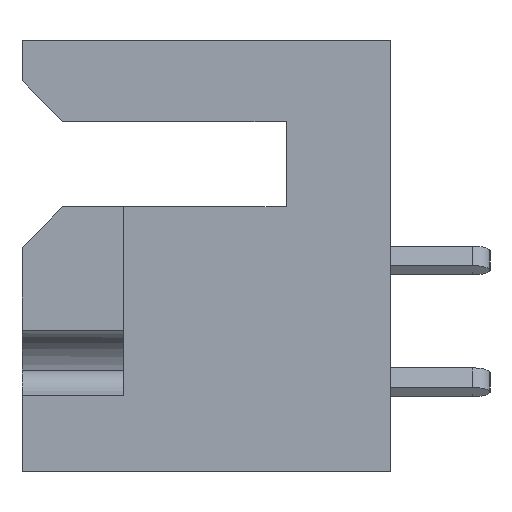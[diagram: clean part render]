
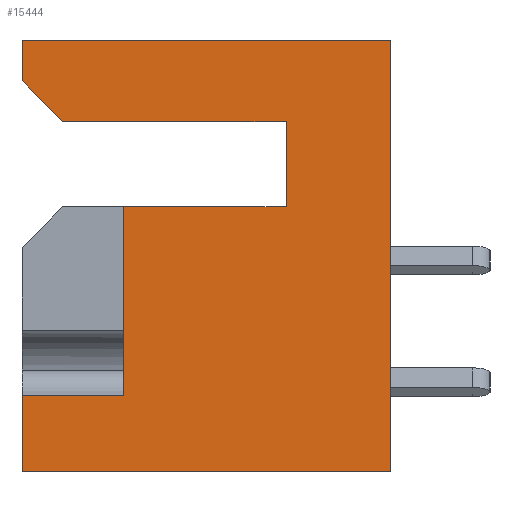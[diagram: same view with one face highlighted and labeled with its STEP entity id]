
A CAD part, left-side view. The second image highlights one B-rep face of the part: STEP entity #15444.
In plain terms, the highlighted planar face has unit normal (-1, 0, 0).
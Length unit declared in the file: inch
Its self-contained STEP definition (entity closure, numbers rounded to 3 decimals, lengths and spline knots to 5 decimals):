
#153 = CARTESIAN_POINT ( 'NONE',  ( 0., 0., 0. ) ) ;
#280 = VERTEX_POINT ( 'NONE', #9337 ) ;
#1365 = ORIENTED_EDGE ( 'NONE', *, *, #15396, .T. ) ;
#1525 = EDGE_CURVE ( 'NONE', #18930, #14563, #5102, .T. ) ;
#1889 = LINE ( 'NONE', #9888, #2685 ) ;
#1892 = DIRECTION ( 'NONE',  ( 0., 0., 1. ) ) ;
#1954 = CARTESIAN_POINT ( 'NONE',  ( 0., 0.453, -0.05 ) ) ;
#2631 = ORIENTED_EDGE ( 'NONE', *, *, #9055, .F. ) ;
#2685 = VECTOR ( 'NONE', #13430, 39.37008 ) ;
#3004 = EDGE_CURVE ( 'NONE', #19937, #14563, #5015, .T. ) ;
#3247 = ORIENTED_EDGE ( 'NONE', *, *, #4225, .T. ) ;
#3399 = VECTOR ( 'NONE', #12668, 39.37008 ) ;
#3476 = CARTESIAN_POINT ( 'NONE',  ( 0., 0.453, 0. ) ) ;
#3514 = VERTEX_POINT ( 'NONE', #11496 ) ;
#3757 = EDGE_CURVE ( 'NONE', #19839, #280, #19363, .T. ) ;
#4225 = EDGE_CURVE ( 'NONE', #7790, #280, #14699, .T. ) ;
#4655 = FACE_OUTER_BOUND ( 'NONE', #16675, .T. ) ;
#4663 = DIRECTION ( 'NONE',  ( 0., 1., 0. ) ) ;
#4704 = CARTESIAN_POINT ( 'NONE',  ( 0., 0.453, 0. ) ) ;
#4725 = CARTESIAN_POINT ( 'NONE',  ( 0., 0.403, -0.1 ) ) ;
#4960 = LINE ( 'NONE', #5603, #15727 ) ;
#5015 = LINE ( 'NONE', #21272, #3399 ) ;
#5102 = LINE ( 'NONE', #19790, #5362 ) ;
#5362 = VECTOR ( 'NONE', #7865, 39.37008 ) ;
#5603 = CARTESIAN_POINT ( 'NONE',  ( 0., 0.128, -0.1 ) ) ;
#6120 = DIRECTION ( 'NONE',  ( 0., -1., 0. ) ) ;
#6795 = LINE ( 'NONE', #9877, #8405 ) ;
#6833 = VECTOR ( 'NONE', #1892, 39.37008 ) ;
#6944 = CARTESIAN_POINT ( 'NONE',  ( 0., 0.453, -0.531 ) ) ;
#7030 = CARTESIAN_POINT ( 'NONE',  ( 0., 0.453, 0. ) ) ;
#7553 = EDGE_CURVE ( 'NONE', #3514, #9352, #6795, .T. ) ;
#7790 = VERTEX_POINT ( 'NONE', #1954 ) ;
#7865 = DIRECTION ( 'NONE',  ( 0., 1., 0. ) ) ;
#8010 = EDGE_CURVE ( 'NONE', #9942, #9390, #18910, .T. ) ;
#8132 = VECTOR ( 'NONE', #12134, 39.37008 ) ;
#8174 = DIRECTION ( 'NONE',  ( 0., -0.707, -0.707 ) ) ;
#8405 = VECTOR ( 'NONE', #4663, 39.37008 ) ;
#8729 = CARTESIAN_POINT ( 'NONE',  ( 0., 0.128, -0.1 ) ) ;
#8762 = AXIS2_PLACEMENT_3D ( 'NONE', #3476, #10390, #20841 ) ;
#8826 = CARTESIAN_POINT ( 'NONE',  ( 0., 0.453, -0.531 ) ) ;
#8922 = CARTESIAN_POINT ( 'NONE',  ( 0., 0., 0. ) ) ;
#9055 = EDGE_CURVE ( 'NONE', #18930, #9352, #1889, .T. ) ;
#9337 = CARTESIAN_POINT ( 'NONE',  ( 0., 0.403, -0.1 ) ) ;
#9352 = VERTEX_POINT ( 'NONE', #10424 ) ;
#9390 = VERTEX_POINT ( 'NONE', #153 ) ;
#9877 = CARTESIAN_POINT ( 'NONE',  ( 0., 0.128, -0.205 ) ) ;
#9888 = CARTESIAN_POINT ( 'NONE',  ( 0., 0.328, -0.205 ) ) ;
#9942 = VERTEX_POINT ( 'NONE', #7030 ) ;
#10118 = EDGE_CURVE ( 'NONE', #22083, #9390, #18016, .T. ) ;
#10214 = ORIENTED_EDGE ( 'NONE', *, *, #10118, .T. ) ;
#10390 = DIRECTION ( 'NONE',  ( 1., 0., 0. ) ) ;
#10424 = CARTESIAN_POINT ( 'NONE',  ( 0., 0.328, -0.205 ) ) ;
#10634 = DIRECTION ( 'NONE',  ( 0., 0., 1. ) ) ;
#10882 = LINE ( 'NONE', #17322, #6833 ) ;
#11025 = ORIENTED_EDGE ( 'NONE', *, *, #12817, .F. ) ;
#11496 = CARTESIAN_POINT ( 'NONE',  ( 0., 0.128, -0.205 ) ) ;
#11565 = ORIENTED_EDGE ( 'NONE', *, *, #1525, .T. ) ;
#12134 = DIRECTION ( 'NONE',  ( 0., -1., 0. ) ) ;
#12335 = VECTOR ( 'NONE', #10634, 39.37008 ) ;
#12504 = EDGE_CURVE ( 'NONE', #3514, #19839, #4960, .T. ) ;
#12668 = DIRECTION ( 'NONE',  ( 0., 0., 1. ) ) ;
#12817 = EDGE_CURVE ( 'NONE', #7790, #9942, #10882, .T. ) ;
#13430 = DIRECTION ( 'NONE',  ( 0., 0., 1. ) ) ;
#13858 = PLANE ( 'NONE',  #8762 ) ;
#13949 = DIRECTION ( 'NONE',  ( 0., 0., 1. ) ) ;
#14049 = LINE ( 'NONE', #8826, #8132 ) ;
#14563 = VERTEX_POINT ( 'NONE', #22109 ) ;
#14699 = LINE ( 'NONE', #4725, #19025 ) ;
#15208 = CARTESIAN_POINT ( 'NONE',  ( 0., 0.128, -0.1 ) ) ;
#15396 = EDGE_CURVE ( 'NONE', #19937, #22083, #14049, .T. ) ;
#15444 = ADVANCED_FACE ( 'NONE', ( #4655 ), #13858, .F. ) ;
#15639 = ORIENTED_EDGE ( 'NONE', *, *, #3757, .F. ) ;
#15727 = VECTOR ( 'NONE', #13949, 39.37008 ) ;
#15954 = ORIENTED_EDGE ( 'NONE', *, *, #8010, .F. ) ;
#16675 = EDGE_LOOP ( 'NONE', ( #11565, #21363, #1365, #10214, #15954, #11025, #3247, #15639, #21538, #16856, #2631 ) ) ;
#16854 = CARTESIAN_POINT ( 'NONE',  ( 0., 0.328, -0.437 ) ) ;
#16856 = ORIENTED_EDGE ( 'NONE', *, *, #7553, .T. ) ;
#17322 = CARTESIAN_POINT ( 'NONE',  ( 0., 0.453, 0. ) ) ;
#18016 = LINE ( 'NONE', #8922, #12335 ) ;
#18360 = VECTOR ( 'NONE', #6120, 39.37008 ) ;
#18808 = CARTESIAN_POINT ( 'NONE',  ( 0., 0., -0.531 ) ) ;
#18910 = LINE ( 'NONE', #4704, #18360 ) ;
#18930 = VERTEX_POINT ( 'NONE', #16854 ) ;
#19025 = VECTOR ( 'NONE', #8174, 39.37008 ) ;
#19121 = DIRECTION ( 'NONE',  ( 0., 1., 0. ) ) ;
#19363 = LINE ( 'NONE', #8729, #21244 ) ;
#19790 = CARTESIAN_POINT ( 'NONE',  ( 0., 0.328, -0.437 ) ) ;
#19839 = VERTEX_POINT ( 'NONE', #15208 ) ;
#19937 = VERTEX_POINT ( 'NONE', #6944 ) ;
#20841 = DIRECTION ( 'NONE',  ( 0., 0., -1. ) ) ;
#21244 = VECTOR ( 'NONE', #19121, 39.37008 ) ;
#21272 = CARTESIAN_POINT ( 'NONE',  ( 0., 0.453, 0. ) ) ;
#21363 = ORIENTED_EDGE ( 'NONE', *, *, #3004, .F. ) ;
#21538 = ORIENTED_EDGE ( 'NONE', *, *, #12504, .F. ) ;
#22083 = VERTEX_POINT ( 'NONE', #18808 ) ;
#22109 = CARTESIAN_POINT ( 'NONE',  ( 0., 0.453, -0.437 ) ) ;
